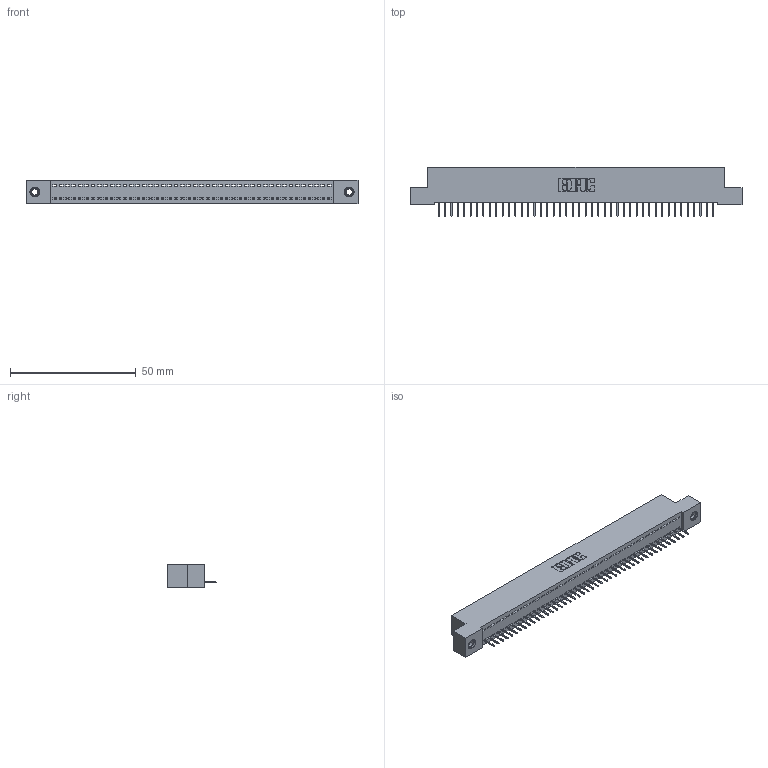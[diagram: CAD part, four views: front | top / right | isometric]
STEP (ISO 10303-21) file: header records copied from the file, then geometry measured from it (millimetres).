
FILE_DESCRIPTION (( 'STEP AP203' ), '1' );
FILE_NAME ('342-044-524-107.STEP', '2019-10-02T19:05:46', ( '' ), ( '' ), 'SwSTEP 2.0', 'SolidWorks 2016', '' );
FILE_SCHEMA (( 'CONFIG_CONTROL_DESIGN' ));
Length unit declared in the file: inch
Products named in the file (4): 342-044-524-107; 342 Part_TI; 345-292-001_345-293-124; 345-250-001_345-250-005-103
Assembly tree (47 placements, depth 2):
  342-044-524-107
    342 Part_TI
    345-292-001_345-293-124  x44
    345-250-001_345-250-005-103  x2
Bounding box: 132.08 x 19.69 x 9.4 mm (x, y, z)
Volume: 11401.6 mm3; surface area: 16272.5 mm2
Topology: 47 solids, 47 shells, 2898 faces, 8355 edges, 5386 vertices
Faces by surface type: plane 2210, cylinder 672, cone 12, torus 4
Entity records: 27768 total; most frequent: CARTESIAN_POINT 4769, ORIENTED_EDGE 4742, DIRECTION 4053, EDGE_CURVE 2371, LINE 2227, VECTOR 2227, VERTEX_POINT 1572, AXIS2_PLACEMENT_3D 913
